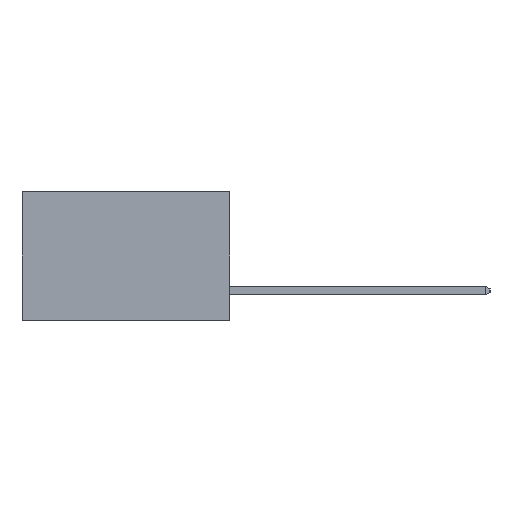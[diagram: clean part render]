
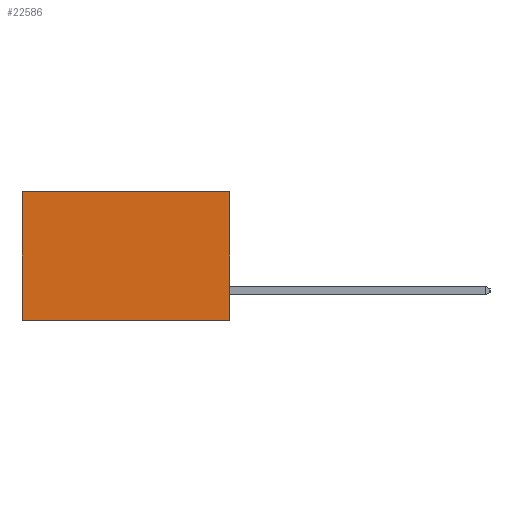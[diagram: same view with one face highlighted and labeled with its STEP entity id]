
A CAD part, left-side view. The second image highlights one B-rep face of the part: STEP entity #22586.
In plain terms, the highlighted planar face has unit normal (-1, 0, 0).
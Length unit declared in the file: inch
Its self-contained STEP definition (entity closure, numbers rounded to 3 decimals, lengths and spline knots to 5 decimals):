
#721 = VECTOR ( 'NONE', #2511, 39.37008 ) ;
#1365 = ORIENTED_EDGE ( 'NONE', *, *, #3813, .T. ) ;
#2175 = CARTESIAN_POINT ( 'NONE',  ( 0.298, 0., 0. ) ) ;
#2511 = DIRECTION ( 'NONE',  ( 0., 0., -1. ) ) ;
#2877 = DIRECTION ( 'NONE',  ( 0., 0., -1. ) ) ;
#3813 = EDGE_CURVE ( 'NONE', #20603, #21245, #11572, .T. ) ;
#5192 = CARTESIAN_POINT ( 'NONE',  ( 0.298, 0., 0. ) ) ;
#6373 = LINE ( 'NONE', #11910, #721 ) ;
#7851 = DIRECTION ( 'NONE',  ( 0., 0., -1. ) ) ;
#8105 = VECTOR ( 'NONE', #21981, 39.37008 ) ;
#8308 = ORIENTED_EDGE ( 'NONE', *, *, #12998, .T. ) ;
#8970 = CARTESIAN_POINT ( 'NONE',  ( 0.298, 0.6, 0. ) ) ;
#10241 = ORIENTED_EDGE ( 'NONE', *, *, #22989, .F. ) ;
#10617 = VERTEX_POINT ( 'NONE', #5192 ) ;
#11572 = LINE ( 'NONE', #8970, #20229 ) ;
#11910 = CARTESIAN_POINT ( 'NONE',  ( 0.298, 0., 0. ) ) ;
#12759 = CARTESIAN_POINT ( 'NONE',  ( 0.298, 0., 0. ) ) ;
#12770 = CARTESIAN_POINT ( 'NONE',  ( 0.298, 0., -0.37 ) ) ;
#12983 = VECTOR ( 'NONE', #16537, 39.37008 ) ;
#12998 = EDGE_CURVE ( 'NONE', #10617, #20603, #17909, .T. ) ;
#13441 = PLANE ( 'NONE',  #24060 ) ;
#13854 = EDGE_LOOP ( 'NONE', ( #1365, #10241, #24090, #8308 ) ) ;
#14879 = LINE ( 'NONE', #12770, #8105 ) ;
#14887 = CARTESIAN_POINT ( 'NONE',  ( 0.298, 0., -0.37 ) ) ;
#15078 = VERTEX_POINT ( 'NONE', #14887 ) ;
#16537 = DIRECTION ( 'NONE',  ( 0., 1., 0. ) ) ;
#17909 = LINE ( 'NONE', #12759, #12983 ) ;
#18046 = FACE_OUTER_BOUND ( 'NONE', #13854, .T. ) ;
#18881 = CARTESIAN_POINT ( 'NONE',  ( 0.298, 0.6, -0.37 ) ) ;
#18977 = DIRECTION ( 'NONE',  ( 1., 0., 0. ) ) ;
#20229 = VECTOR ( 'NONE', #2877, 39.37008 ) ;
#20461 = CARTESIAN_POINT ( 'NONE',  ( 0.298, 0.6, 0. ) ) ;
#20603 = VERTEX_POINT ( 'NONE', #20461 ) ;
#21245 = VERTEX_POINT ( 'NONE', #18881 ) ;
#21981 = DIRECTION ( 'NONE',  ( 0., 1., 0. ) ) ;
#22586 = ADVANCED_FACE ( 'NONE', ( #18046 ), #13441, .F. ) ;
#22695 = EDGE_CURVE ( 'NONE', #10617, #15078, #6373, .T. ) ;
#22989 = EDGE_CURVE ( 'NONE', #15078, #21245, #14879, .T. ) ;
#24060 = AXIS2_PLACEMENT_3D ( 'NONE', #2175, #18977, #7851 ) ;
#24090 = ORIENTED_EDGE ( 'NONE', *, *, #22695, .F. ) ;
